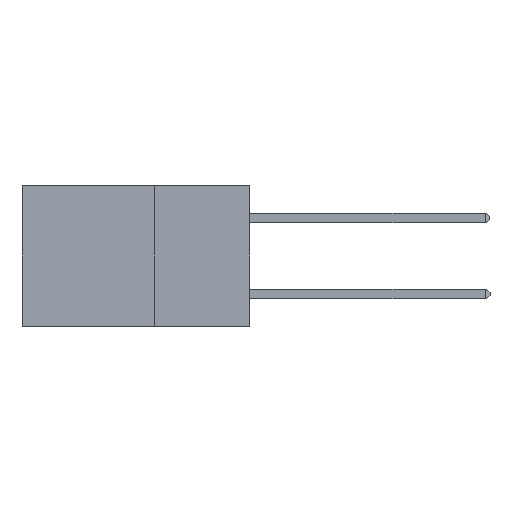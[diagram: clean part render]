
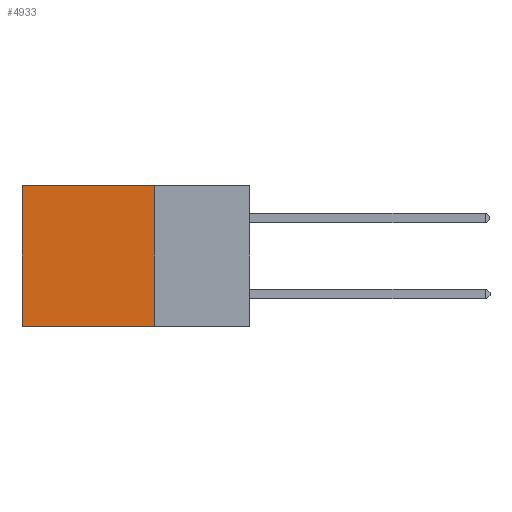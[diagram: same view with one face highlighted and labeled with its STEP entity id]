
A CAD part, left-side view. The second image highlights one B-rep face of the part: STEP entity #4933.
In plain terms, the highlighted planar face has unit normal (-1, 0, 0).
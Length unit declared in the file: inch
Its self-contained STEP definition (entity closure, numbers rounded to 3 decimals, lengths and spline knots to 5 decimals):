
#57 = VERTEX_POINT ( 'NONE', #8356 ) ;
#108 = DIRECTION ( 'NONE',  ( 0., 1., 0. ) ) ;
#552 = DIRECTION ( 'NONE',  ( 0., 0., -1. ) ) ;
#570 = DIRECTION ( 'NONE',  ( 0., 1., 0. ) ) ;
#785 = EDGE_CURVE ( 'NONE', #57, #11427, #2693, .T. ) ;
#1837 = AXIS2_PLACEMENT_3D ( 'NONE', #11575, #4573, #14294 ) ;
#2329 = LINE ( 'NONE', #7176, #16158 ) ;
#2693 = LINE ( 'NONE', #7300, #9714 ) ;
#3185 = VERTEX_POINT ( 'NONE', #9760 ) ;
#3876 = VECTOR ( 'NONE', #552, 39.37008 ) ;
#4573 = DIRECTION ( 'NONE',  ( 1., 0., 0. ) ) ;
#4933 = ADVANCED_FACE ( 'NONE', ( #14324 ), #12924, .F. ) ;
#5492 = EDGE_CURVE ( 'NONE', #16463, #57, #2329, .T. ) ;
#5630 = EDGE_CURVE ( 'NONE', #16463, #3185, #7142, .T. ) ;
#7069 = VECTOR ( 'NONE', #570, 39.37008 ) ;
#7142 = LINE ( 'NONE', #9008, #3876 ) ;
#7176 = CARTESIAN_POINT ( 'NONE',  ( 0.2875, 0.25, 0. ) ) ;
#7300 = CARTESIAN_POINT ( 'NONE',  ( 0.2875, 0.6, 0. ) ) ;
#8356 = CARTESIAN_POINT ( 'NONE',  ( 0.2875, 0.6, 0. ) ) ;
#8708 = DIRECTION ( 'NONE',  ( 0., 0., -1. ) ) ;
#8968 = CARTESIAN_POINT ( 'NONE',  ( 0.2875, 0.25, -0.37 ) ) ;
#9008 = CARTESIAN_POINT ( 'NONE',  ( 0.2875, 0.25, 0. ) ) ;
#9714 = VECTOR ( 'NONE', #8708, 39.37008 ) ;
#9760 = CARTESIAN_POINT ( 'NONE',  ( 0.2875, 0.25, -0.37 ) ) ;
#10814 = LINE ( 'NONE', #8968, #7069 ) ;
#11427 = VERTEX_POINT ( 'NONE', #15731 ) ;
#11575 = CARTESIAN_POINT ( 'NONE',  ( 0.2875, 0.25, 0. ) ) ;
#12069 = EDGE_LOOP ( 'NONE', ( #17277, #17673, #12376, #16385 ) ) ;
#12376 = ORIENTED_EDGE ( 'NONE', *, *, #5630, .F. ) ;
#12924 = PLANE ( 'NONE',  #1837 ) ;
#14294 = DIRECTION ( 'NONE',  ( 0., 0., -1. ) ) ;
#14324 = FACE_OUTER_BOUND ( 'NONE', #12069, .T. ) ;
#15731 = CARTESIAN_POINT ( 'NONE',  ( 0.2875, 0.6, -0.37 ) ) ;
#16158 = VECTOR ( 'NONE', #108, 39.37008 ) ;
#16385 = ORIENTED_EDGE ( 'NONE', *, *, #5492, .T. ) ;
#16463 = VERTEX_POINT ( 'NONE', #17052 ) ;
#16485 = EDGE_CURVE ( 'NONE', #3185, #11427, #10814, .T. ) ;
#17052 = CARTESIAN_POINT ( 'NONE',  ( 0.2875, 0.25, 0. ) ) ;
#17277 = ORIENTED_EDGE ( 'NONE', *, *, #785, .T. ) ;
#17673 = ORIENTED_EDGE ( 'NONE', *, *, #16485, .F. ) ;
